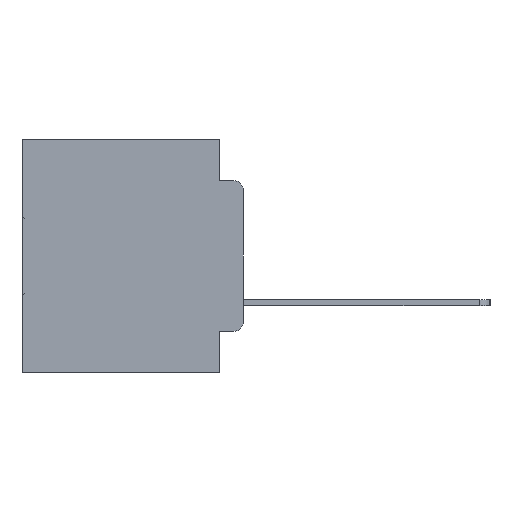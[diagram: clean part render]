
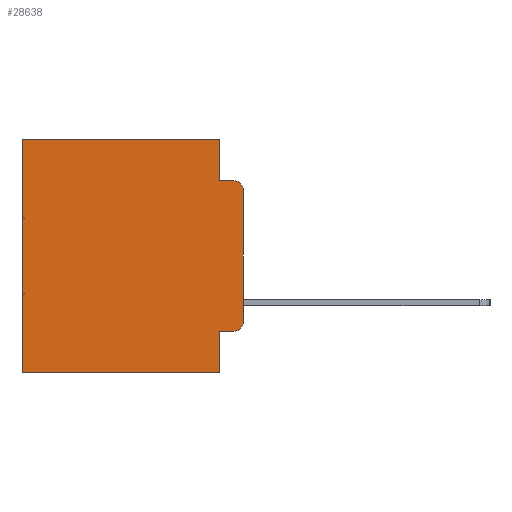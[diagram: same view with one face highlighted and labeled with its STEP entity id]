
A CAD part, left-side view. The second image highlights one B-rep face of the part: STEP entity #28638.
In plain terms, the highlighted planar face has unit normal (-1, 0, 0).
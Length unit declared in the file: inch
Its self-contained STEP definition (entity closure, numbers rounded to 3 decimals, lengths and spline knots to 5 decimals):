
#155 = VERTEX_POINT ( 'NONE', #17816 ) ;
#332 = DIRECTION ( 'NONE',  ( 0., 0., -1. ) ) ;
#550 = DIRECTION ( 'NONE',  ( 0., 0., -1. ) ) ;
#4236 = ORIENTED_EDGE ( 'NONE', *, *, #18854, .F. ) ;
#4322 = VERTEX_POINT ( 'NONE', #12405 ) ;
#5334 = VERTEX_POINT ( 'NONE', #26085 ) ;
#5343 = VERTEX_POINT ( 'NONE', #28453 ) ;
#5454 = VERTEX_POINT ( 'NONE', #6179 ) ;
#5856 = LINE ( 'NONE', #8561, #25494 ) ;
#6179 = CARTESIAN_POINT ( 'NONE',  ( 0.298, 0.02, -0.0885 ) ) ;
#6214 = VECTOR ( 'NONE', #550, 39.37008 ) ;
#7330 = CARTESIAN_POINT ( 'NONE',  ( 0.298, 0.473, 0. ) ) ;
#7374 = AXIS2_PLACEMENT_3D ( 'NONE', #30018, #15029, #32512 ) ;
#7468 = EDGE_CURVE ( 'NONE', #155, #8127, #17121, .T. ) ;
#8127 = VERTEX_POINT ( 'NONE', #17412 ) ;
#8257 = CARTESIAN_POINT ( 'NONE',  ( 0.298, 0.02, -0.3915 ) ) ;
#8282 = EDGE_CURVE ( 'NONE', #25152, #5454, #26049, .T. ) ;
#8561 = CARTESIAN_POINT ( 'NONE',  ( 0.298, 0.051, -0.0885 ) ) ;
#8892 = CARTESIAN_POINT ( 'NONE',  ( 0.298, 0., -0.5 ) ) ;
#9758 = AXIS2_PLACEMENT_3D ( 'NONE', #8257, #26050, #10889 ) ;
#9843 = LINE ( 'NONE', #31125, #15920 ) ;
#10461 = ORIENTED_EDGE ( 'NONE', *, *, #16201, .T. ) ;
#10706 = VECTOR ( 'NONE', #20668, 39.37008 ) ;
#10889 = DIRECTION ( 'NONE',  ( 0., 0., -1. ) ) ;
#11331 = EDGE_CURVE ( 'NONE', #5343, #5454, #5856, .T. ) ;
#11374 = CARTESIAN_POINT ( 'NONE',  ( 0.298, 0., -0.1085 ) ) ;
#11588 = CARTESIAN_POINT ( 'NONE',  ( 0.298, 0.051, -0.4115 ) ) ;
#11689 = VERTEX_POINT ( 'NONE', #27608 ) ;
#11811 = PLANE ( 'NONE',  #29192 ) ;
#12405 = CARTESIAN_POINT ( 'NONE',  ( 0.298, 0.051, -0.5 ) ) ;
#12524 = ORIENTED_EDGE ( 'NONE', *, *, #8282, .T. ) ;
#12886 = VECTOR ( 'NONE', #332, 39.37008 ) ;
#13209 = EDGE_CURVE ( 'NONE', #5334, #11689, #9843, .T. ) ;
#13234 = LINE ( 'NONE', #23940, #6214 ) ;
#13480 = DIRECTION ( 'NONE',  ( 0., 1., 0. ) ) ;
#13760 = ORIENTED_EDGE ( 'NONE', *, *, #17898, .F. ) ;
#15029 = DIRECTION ( 'NONE',  ( -1., 0., 0. ) ) ;
#15376 = ORIENTED_EDGE ( 'NONE', *, *, #23915, .F. ) ;
#15920 = VECTOR ( 'NONE', #13480, 39.37008 ) ;
#16201 = EDGE_CURVE ( 'NONE', #8127, #26713, #32118, .T. ) ;
#16388 = DIRECTION ( 'NONE',  ( 0., -1., 0. ) ) ;
#16995 = DIRECTION ( 'NONE',  ( 0., 0., -1. ) ) ;
#17121 = LINE ( 'NONE', #11588, #29595 ) ;
#17352 = ORIENTED_EDGE ( 'NONE', *, *, #11331, .F. ) ;
#17412 = CARTESIAN_POINT ( 'NONE',  ( 0.298, 0.02, -0.4115 ) ) ;
#17555 = LINE ( 'NONE', #25654, #10706 ) ;
#17816 = CARTESIAN_POINT ( 'NONE',  ( 0.298, 0.051, -0.4115 ) ) ;
#17898 = EDGE_CURVE ( 'NONE', #155, #4322, #13234, .T. ) ;
#18428 = VECTOR ( 'NONE', #21650, 39.37008 ) ;
#18854 = EDGE_CURVE ( 'NONE', #5334, #5343, #17555, .T. ) ;
#19219 = LINE ( 'NONE', #8892, #18428 ) ;
#20452 = LINE ( 'NONE', #31165, #12886 ) ;
#20668 = DIRECTION ( 'NONE',  ( 0., 0., -1. ) ) ;
#20891 = ORIENTED_EDGE ( 'NONE', *, *, #23254, .F. ) ;
#21650 = DIRECTION ( 'NONE',  ( 0., 1., 0. ) ) ;
#21809 = CARTESIAN_POINT ( 'NONE',  ( 0.298, 0., 0. ) ) ;
#22388 = LINE ( 'NONE', #7330, #26673 ) ;
#22880 = FACE_OUTER_BOUND ( 'NONE', #25036, .T. ) ;
#22999 = EDGE_CURVE ( 'NONE', #11689, #29516, #22388, .T. ) ;
#23254 = EDGE_CURVE ( 'NONE', #25152, #26713, #20452, .T. ) ;
#23611 = ORIENTED_EDGE ( 'NONE', *, *, #7468, .T. ) ;
#23915 = EDGE_CURVE ( 'NONE', #4322, #29516, #19219, .T. ) ;
#23940 = CARTESIAN_POINT ( 'NONE',  ( 0.298, 0.051, 0. ) ) ;
#23984 = ORIENTED_EDGE ( 'NONE', *, *, #13209, .T. ) ;
#25036 = EDGE_LOOP ( 'NONE', ( #20891, #12524, #17352, #4236, #23984, #31410, #15376, #13760, #23611, #10461 ) ) ;
#25152 = VERTEX_POINT ( 'NONE', #11374 ) ;
#25494 = VECTOR ( 'NONE', #16388, 39.37008 ) ;
#25654 = CARTESIAN_POINT ( 'NONE',  ( 0.298, 0.051, 0. ) ) ;
#26049 = CIRCLE ( 'NONE', #7374, 0.02 ) ;
#26050 = DIRECTION ( 'NONE',  ( -1., 0., 0. ) ) ;
#26085 = CARTESIAN_POINT ( 'NONE',  ( 0.298, 0.051, 0. ) ) ;
#26673 = VECTOR ( 'NONE', #27681, 39.37008 ) ;
#26713 = VERTEX_POINT ( 'NONE', #32832 ) ;
#27608 = CARTESIAN_POINT ( 'NONE',  ( 0.298, 0.473, 0. ) ) ;
#27681 = DIRECTION ( 'NONE',  ( 0., 0., -1. ) ) ;
#27840 = CARTESIAN_POINT ( 'NONE',  ( 0.298, 0.473, -0.5 ) ) ;
#28453 = CARTESIAN_POINT ( 'NONE',  ( 0.298, 0.051, -0.0885 ) ) ;
#28638 = ADVANCED_FACE ( 'NONE', ( #22880 ), #11811, .F. ) ;
#29192 = AXIS2_PLACEMENT_3D ( 'NONE', #21809, #31930, #16995 ) ;
#29199 = DIRECTION ( 'NONE',  ( 0., -1., 0. ) ) ;
#29516 = VERTEX_POINT ( 'NONE', #27840 ) ;
#29595 = VECTOR ( 'NONE', #29199, 39.37008 ) ;
#30018 = CARTESIAN_POINT ( 'NONE',  ( 0.298, 0.02, -0.1085 ) ) ;
#31125 = CARTESIAN_POINT ( 'NONE',  ( 0.298, 0., 0. ) ) ;
#31165 = CARTESIAN_POINT ( 'NONE',  ( 0.298, 0., 0. ) ) ;
#31410 = ORIENTED_EDGE ( 'NONE', *, *, #22999, .T. ) ;
#31930 = DIRECTION ( 'NONE',  ( 1., 0., 0. ) ) ;
#32118 = CIRCLE ( 'NONE', #9758, 0.02 ) ;
#32512 = DIRECTION ( 'NONE',  ( 0., 0., -1. ) ) ;
#32832 = CARTESIAN_POINT ( 'NONE',  ( 0.298, 0., -0.3915 ) ) ;
